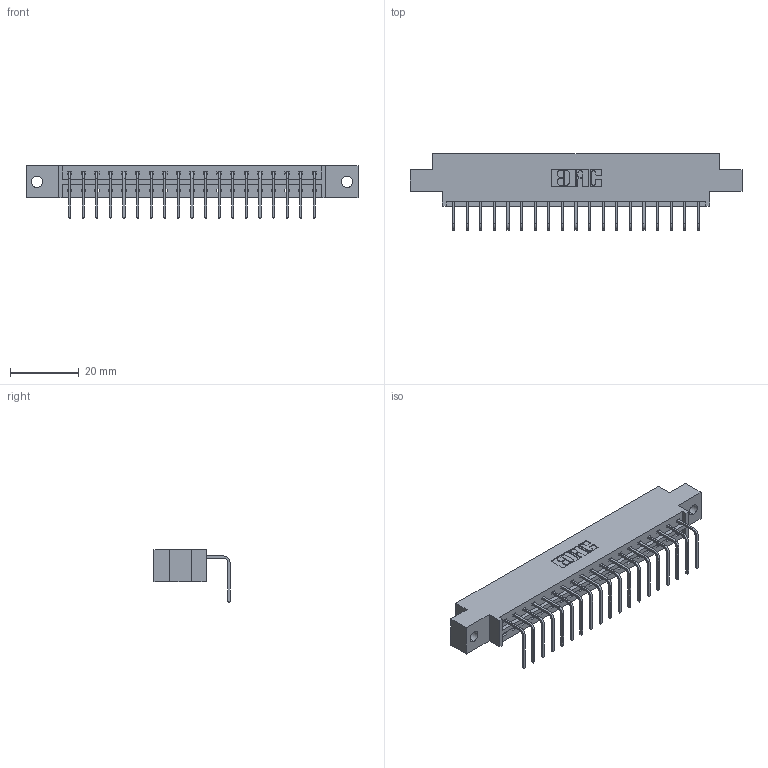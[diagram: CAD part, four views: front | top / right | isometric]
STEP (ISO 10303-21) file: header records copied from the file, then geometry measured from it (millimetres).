
FILE_DESCRIPTION (( 'STEP AP203' ), '1' );
FILE_NAME ('333-019-558-602.STEP', '2018-08-01T23:24:39', ( '' ), ( '' ), 'SwSTEP 2.0', 'SolidWorks 2016', '' );
FILE_SCHEMA (( 'CONFIG_CONTROL_DESIGN' ));
Length unit declared in the file: inch
Products named in the file (3): 333 Part_Offset - .128 Dia; 345-292-001_558 Tail - 2; 333-019-558-602
Assembly tree (20 placements, depth 2):
  333-019-558-602
    333 Part_Offset - .128 Dia
    345-292-001_558 Tail - 2  x19
Bounding box: 96.82 x 22.17 x 15.37 mm (x, y, z)
Volume: 9344.3 mm3; surface area: 10273.8 mm2
Topology: 20 solids, 20 shells, 1258 faces, 3781 edges, 2494 vertices
Faces by surface type: plane 910, cylinder 348
Entity records: 14809 total; most frequent: CARTESIAN_POINT 2567, ORIENTED_EDGE 2522, DIRECTION 2211, EDGE_CURVE 1261, VECTOR 1133, LINE 1133, VERTEX_POINT 838, AXIS2_PLACEMENT_3D 539
